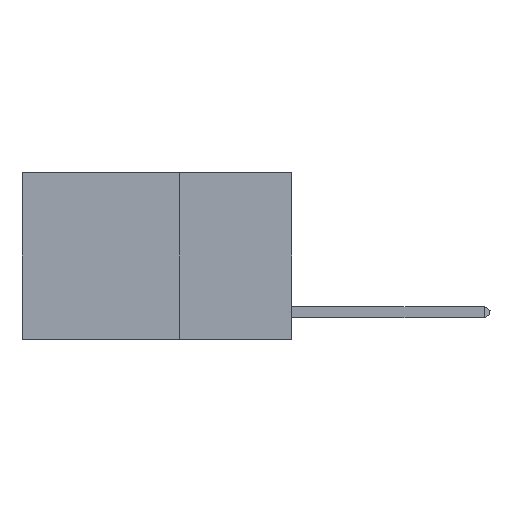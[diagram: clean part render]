
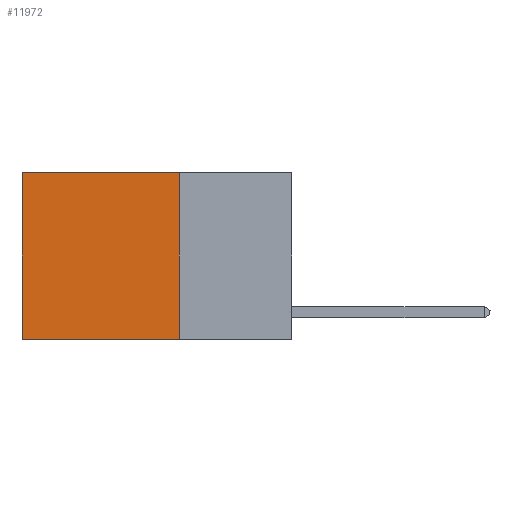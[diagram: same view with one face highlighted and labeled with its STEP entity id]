
A CAD part, left-side view. The second image highlights one B-rep face of the part: STEP entity #11972.
In plain terms, the highlighted planar face has unit normal (-1, 0, 0).
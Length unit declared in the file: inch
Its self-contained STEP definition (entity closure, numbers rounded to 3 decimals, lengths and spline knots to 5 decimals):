
#68 = ORIENTED_EDGE ( 'NONE', *, *, #6345, .T. ) ;
#319 = DIRECTION ( 'NONE',  ( 1., 0., 0. ) ) ;
#660 = CARTESIAN_POINT ( 'NONE',  ( 0.2625, 0.6, 0. ) ) ;
#787 = CARTESIAN_POINT ( 'NONE',  ( 0.2625, 0.6, -0.37 ) ) ;
#881 = DIRECTION ( 'NONE',  ( 0., 1., 0. ) ) ;
#1323 = DIRECTION ( 'NONE',  ( 0., 1., 0. ) ) ;
#1358 = VERTEX_POINT ( 'NONE', #7319 ) ;
#1741 = EDGE_CURVE ( 'NONE', #7044, #1358, #2804, .T. ) ;
#1986 = LINE ( 'NONE', #8473, #10139 ) ;
#2013 = AXIS2_PLACEMENT_3D ( 'NONE', #2239, #319, #7445 ) ;
#2239 = CARTESIAN_POINT ( 'NONE',  ( 0.2625, 0.25, 0. ) ) ;
#2531 = VERTEX_POINT ( 'NONE', #787 ) ;
#2804 = LINE ( 'NONE', #8044, #5192 ) ;
#3056 = ORIENTED_EDGE ( 'NONE', *, *, #12297, .T. ) ;
#3757 = LINE ( 'NONE', #660, #5839 ) ;
#4106 = LINE ( 'NONE', #13079, #11944 ) ;
#5192 = VECTOR ( 'NONE', #10147, 39.37008 ) ;
#5457 = ORIENTED_EDGE ( 'NONE', *, *, #8263, .F. ) ;
#5839 = VECTOR ( 'NONE', #11814, 39.37008 ) ;
#6345 = EDGE_CURVE ( 'NONE', #9305, #2531, #3757, .T. ) ;
#7044 = VERTEX_POINT ( 'NONE', #12074 ) ;
#7107 = CARTESIAN_POINT ( 'NONE',  ( 0.2625, 0.6, 0. ) ) ;
#7319 = CARTESIAN_POINT ( 'NONE',  ( 0.2625, 0.25, -0.37 ) ) ;
#7445 = DIRECTION ( 'NONE',  ( 0., 0., -1. ) ) ;
#7958 = EDGE_LOOP ( 'NONE', ( #68, #5457, #8199, #3056 ) ) ;
#8044 = CARTESIAN_POINT ( 'NONE',  ( 0.2625, 0.25, 0. ) ) ;
#8199 = ORIENTED_EDGE ( 'NONE', *, *, #1741, .F. ) ;
#8263 = EDGE_CURVE ( 'NONE', #1358, #2531, #1986, .T. ) ;
#8473 = CARTESIAN_POINT ( 'NONE',  ( 0.2625, 0.25, -0.37 ) ) ;
#9305 = VERTEX_POINT ( 'NONE', #7107 ) ;
#10139 = VECTOR ( 'NONE', #1323, 39.37008 ) ;
#10147 = DIRECTION ( 'NONE',  ( 0., 0., -1. ) ) ;
#10451 = PLANE ( 'NONE',  #2013 ) ;
#10682 = FACE_OUTER_BOUND ( 'NONE', #7958, .T. ) ;
#11814 = DIRECTION ( 'NONE',  ( 0., 0., -1. ) ) ;
#11944 = VECTOR ( 'NONE', #881, 39.37008 ) ;
#11972 = ADVANCED_FACE ( 'NONE', ( #10682 ), #10451, .F. ) ;
#12074 = CARTESIAN_POINT ( 'NONE',  ( 0.2625, 0.25, 0. ) ) ;
#12297 = EDGE_CURVE ( 'NONE', #7044, #9305, #4106, .T. ) ;
#13079 = CARTESIAN_POINT ( 'NONE',  ( 0.2625, 0.25, 0. ) ) ;
